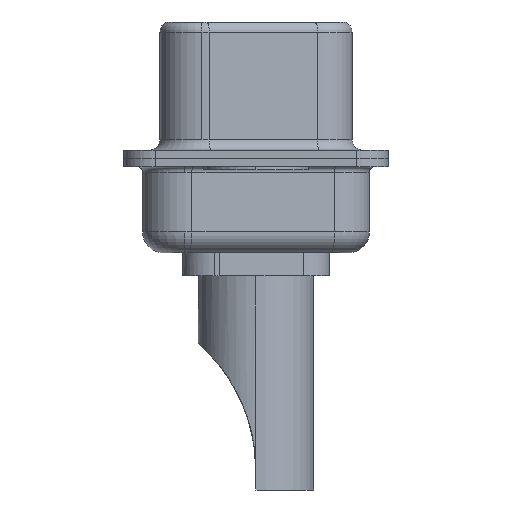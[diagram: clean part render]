
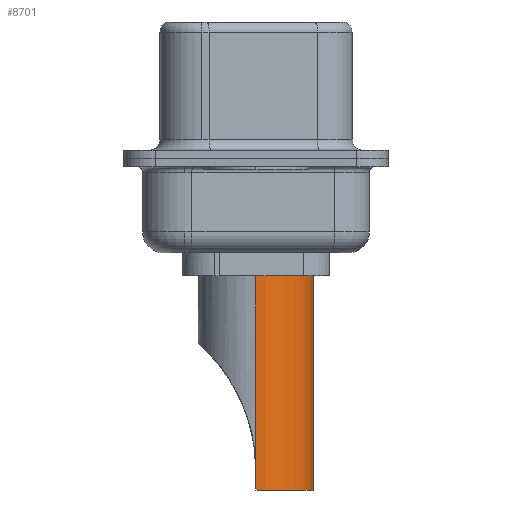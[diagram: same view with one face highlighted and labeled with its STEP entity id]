
A CAD part, left-side view. The second image highlights one B-rep face of the part: STEP entity #8701.
In plain terms, the highlighted cylindrical face has radius 2.75 mm (diameter 5.5 mm), a partial arc.
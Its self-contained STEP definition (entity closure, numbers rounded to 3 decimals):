
#117 = AXIS2_PLACEMENT_3D ( 'NONE', #6387, #8829, #5163 ) ;
#218 = DIRECTION ( 'NONE',  ( 0., 0., 1. ) ) ;
#499 = LINE ( 'NONE', #15498, #6502 ) ;
#1377 = CIRCLE ( 'NONE', #10550, 2.75 ) ;
#1448 = CARTESIAN_POINT ( 'NONE',  ( 0., 0., -8.7 ) ) ;
#1510 = EDGE_CURVE ( 'NONE', #2945, #10906, #12101, .T. ) ;
#1541 = DIRECTION ( 'NONE',  ( 0., 0., 1. ) ) ;
#1637 = CARTESIAN_POINT ( 'NONE',  ( -2.75, 0., -7.764 ) ) ;
#1689 = ORIENTED_EDGE ( 'NONE', *, *, #1510, .T. ) ;
#2117 = CARTESIAN_POINT ( 'NONE',  ( 0., 0., 1.5 ) ) ;
#2681 = DIRECTION ( 'NONE',  ( 1., 0., 0. ) ) ;
#2945 = VERTEX_POINT ( 'NONE', #7336 ) ;
#3523 = CARTESIAN_POINT ( 'NONE',  ( -2.75, 0., -8.7 ) ) ;
#4325 = CARTESIAN_POINT ( 'NONE',  ( 2.75, 0., -8.7 ) ) ;
#5076 = EDGE_CURVE ( 'NONE', #2945, #8859, #499, .T. ) ;
#5085 = ORIENTED_EDGE ( 'NONE', *, *, #5188, .F. ) ;
#5163 = DIRECTION ( 'NONE',  ( 1., 0., 0. ) ) ;
#5188 = EDGE_CURVE ( 'NONE', #8514, #12846, #11447, .T. ) ;
#5383 = EDGE_CURVE ( 'NONE', #12846, #10906, #12364, .T. ) ;
#5653 = VECTOR ( 'NONE', #1541, 1000. ) ;
#6256 = ORIENTED_EDGE ( 'NONE', *, *, #7905, .T. ) ;
#6387 = CARTESIAN_POINT ( 'NONE',  ( 0., 0., 4.234 ) ) ;
#6502 = VECTOR ( 'NONE', #8414, 1000. ) ;
#6593 = CARTESIAN_POINT ( 'NONE',  ( 2.75, 0., 1.5 ) ) ;
#7336 = CARTESIAN_POINT ( 'NONE',  ( 2.75, 0., -7.764 ) ) ;
#7905 = EDGE_CURVE ( 'NONE', #8514, #10807, #9678, .T. ) ;
#7999 = CARTESIAN_POINT ( 'NONE',  ( -2.75, 0., 1.5 ) ) ;
#8180 = ORIENTED_EDGE ( 'NONE', *, *, #5383, .F. ) ;
#8406 = EDGE_LOOP ( 'NONE', ( #5085, #6256, #10631, #11967, #1689, #8180 ) ) ;
#8414 = DIRECTION ( 'NONE',  ( 0., 0., -1. ) ) ;
#8514 = VERTEX_POINT ( 'NONE', #1637 ) ;
#8689 = CYLINDRICAL_SURFACE ( 'NONE', #117, 2.75 ) ;
#8701 = ADVANCED_FACE ( 'NONE', ( #9079 ), #8689, .T. ) ;
#8829 = DIRECTION ( 'NONE',  ( 0., 0., 1. ) ) ;
#8859 = VERTEX_POINT ( 'NONE', #4325 ) ;
#9079 = FACE_OUTER_BOUND ( 'NONE', #8406, .T. ) ;
#9206 = DIRECTION ( 'NONE',  ( 0., 0., 1. ) ) ;
#9678 = LINE ( 'NONE', #3523, #12487 ) ;
#9898 = CARTESIAN_POINT ( 'NONE',  ( -2.75, 0., -8.7 ) ) ;
#9913 = DIRECTION ( 'NONE',  ( 0., 0., 1. ) ) ;
#10550 = AXIS2_PLACEMENT_3D ( 'NONE', #1448, #9913, #2681 ) ;
#10631 = ORIENTED_EDGE ( 'NONE', *, *, #13646, .T. ) ;
#10764 = DIRECTION ( 'NONE',  ( 0., 0., -1. ) ) ;
#10807 = VERTEX_POINT ( 'NONE', #9898 ) ;
#10906 = VERTEX_POINT ( 'NONE', #6593 ) ;
#11447 = LINE ( 'NONE', #14196, #11812 ) ;
#11812 = VECTOR ( 'NONE', #9206, 1000. ) ;
#11967 = ORIENTED_EDGE ( 'NONE', *, *, #5076, .F. ) ;
#12101 = LINE ( 'NONE', #15063, #5653 ) ;
#12364 = CIRCLE ( 'NONE', #14788, 2.75 ) ;
#12487 = VECTOR ( 'NONE', #10764, 1000. ) ;
#12846 = VERTEX_POINT ( 'NONE', #7999 ) ;
#13646 = EDGE_CURVE ( 'NONE', #10807, #8859, #1377, .T. ) ;
#14196 = CARTESIAN_POINT ( 'NONE',  ( -2.75, 0., 4.234 ) ) ;
#14788 = AXIS2_PLACEMENT_3D ( 'NONE', #2117, #218, #14796 ) ;
#14796 = DIRECTION ( 'NONE',  ( 1., 0., 0. ) ) ;
#15063 = CARTESIAN_POINT ( 'NONE',  ( 2.75, 0., 4.234 ) ) ;
#15498 = CARTESIAN_POINT ( 'NONE',  ( 2.75, 0., -8.7 ) ) ;
